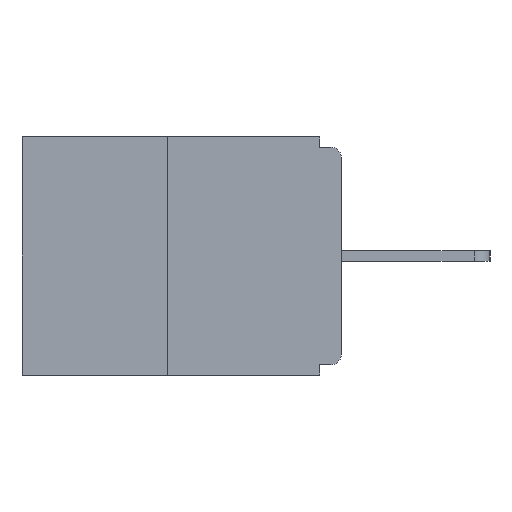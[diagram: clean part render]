
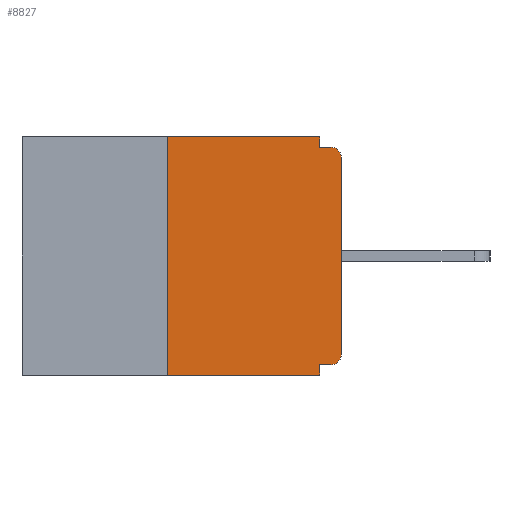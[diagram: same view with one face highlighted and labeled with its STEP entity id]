
A CAD part, left-side view. The second image highlights one B-rep face of the part: STEP entity #8827.
In plain terms, the highlighted planar face has unit normal (-1, 0, 0).
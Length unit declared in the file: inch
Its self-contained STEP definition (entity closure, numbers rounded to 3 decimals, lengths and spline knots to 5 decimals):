
#104 = DIRECTION ( 'NONE',  ( 0., 0., -1. ) ) ;
#195 = CARTESIAN_POINT ( 'NONE',  ( 0., 0.031, -0.343 ) ) ;
#654 = EDGE_CURVE ( 'NONE', #1624, #10731, #8116, .T. ) ;
#824 = EDGE_CURVE ( 'NONE', #11968, #11429, #8155, .T. ) ;
#857 = CARTESIAN_POINT ( 'NONE',  ( 0., 0.46, 0. ) ) ;
#1191 = LINE ( 'NONE', #7887, #2942 ) ;
#1624 = VERTEX_POINT ( 'NONE', #2291 ) ;
#1699 = CARTESIAN_POINT ( 'NONE',  ( 0., 0.031, 0. ) ) ;
#1733 = ORIENTED_EDGE ( 'NONE', *, *, #8710, .T. ) ;
#2024 = DIRECTION ( 'NONE',  ( 0., 0., 1. ) ) ;
#2278 = LINE ( 'NONE', #11873, #8017 ) ;
#2291 = CARTESIAN_POINT ( 'NONE',  ( 0., 0.031, -0.015 ) ) ;
#2858 = DIRECTION ( 'NONE',  ( 0., 0., -1. ) ) ;
#2942 = VECTOR ( 'NONE', #5036, 39.37008 ) ;
#2958 = CARTESIAN_POINT ( 'NONE',  ( 0., 0., -0.015 ) ) ;
#3129 = EDGE_CURVE ( 'NONE', #13975, #12895, #1191, .T. ) ;
#3325 = AXIS2_PLACEMENT_3D ( 'NONE', #9244, #11876, #104 ) ;
#3778 = CARTESIAN_POINT ( 'NONE',  ( 0., 0.015, -0.328 ) ) ;
#3844 = EDGE_CURVE ( 'NONE', #11429, #1624, #8609, .T. ) ;
#4125 = ORIENTED_EDGE ( 'NONE', *, *, #3844, .F. ) ;
#4272 = DIRECTION ( 'NONE',  ( 0., -1., 0. ) ) ;
#4314 = DIRECTION ( 'NONE',  ( 0., -1., 0. ) ) ;
#4321 = LINE ( 'NONE', #195, #10797 ) ;
#4856 = ORIENTED_EDGE ( 'NONE', *, *, #3129, .T. ) ;
#4951 = CIRCLE ( 'NONE', #3325, 0.015 ) ;
#4992 = AXIS2_PLACEMENT_3D ( 'NONE', #12094, #14633, #2858 ) ;
#5036 = DIRECTION ( 'NONE',  ( 0., -1., 0. ) ) ;
#5140 = EDGE_CURVE ( 'NONE', #9505, #16382, #11121, .T. ) ;
#5442 = ORIENTED_EDGE ( 'NONE', *, *, #10091, .F. ) ;
#5775 = DIRECTION ( 'NONE',  ( 0., 0., -1. ) ) ;
#5780 = CARTESIAN_POINT ( 'NONE',  ( 0., 0.25, -0.343 ) ) ;
#5979 = CARTESIAN_POINT ( 'NONE',  ( 0., 0.031, -0.343 ) ) ;
#6184 = ORIENTED_EDGE ( 'NONE', *, *, #6831, .F. ) ;
#6249 = DIRECTION ( 'NONE',  ( 0., 0., 1. ) ) ;
#6585 = VECTOR ( 'NONE', #2024, 39.37008 ) ;
#6831 = EDGE_CURVE ( 'NONE', #7837, #9933, #2278, .T. ) ;
#7065 = CARTESIAN_POINT ( 'NONE',  ( 0., 0.25, 0. ) ) ;
#7837 = VERTEX_POINT ( 'NONE', #3778 ) ;
#7887 = CARTESIAN_POINT ( 'NONE',  ( 0., 0.46, -0.343 ) ) ;
#8017 = VECTOR ( 'NONE', #8023, 39.37008 ) ;
#8023 = DIRECTION ( 'NONE',  ( 0., 1., 0. ) ) ;
#8116 = LINE ( 'NONE', #2958, #9184 ) ;
#8155 = LINE ( 'NONE', #14136, #13614 ) ;
#8609 = LINE ( 'NONE', #15327, #10769 ) ;
#8710 = EDGE_CURVE ( 'NONE', #16382, #10731, #13024, .T. ) ;
#8827 = ADVANCED_FACE ( 'NONE', ( #12708 ), #15400, .F. ) ;
#8839 = CARTESIAN_POINT ( 'NONE',  ( 0., 0.25, 0. ) ) ;
#8859 = ORIENTED_EDGE ( 'NONE', *, *, #654, .F. ) ;
#9184 = VECTOR ( 'NONE', #4314, 39.37008 ) ;
#9244 = CARTESIAN_POINT ( 'NONE',  ( 0., 0.015, -0.313 ) ) ;
#9505 = VERTEX_POINT ( 'NONE', #9589 ) ;
#9589 = CARTESIAN_POINT ( 'NONE',  ( 0., 0., -0.313 ) ) ;
#9782 = ORIENTED_EDGE ( 'NONE', *, *, #11628, .T. ) ;
#9933 = VERTEX_POINT ( 'NONE', #14328 ) ;
#10091 = EDGE_CURVE ( 'NONE', #9933, #12895, #4321, .T. ) ;
#10225 = LINE ( 'NONE', #8839, #13566 ) ;
#10244 = AXIS2_PLACEMENT_3D ( 'NONE', #857, #16616, #11095 ) ;
#10671 = ORIENTED_EDGE ( 'NONE', *, *, #824, .F. ) ;
#10731 = VERTEX_POINT ( 'NONE', #12472 ) ;
#10769 = VECTOR ( 'NONE', #15154, 39.37008 ) ;
#10797 = VECTOR ( 'NONE', #5775, 39.37008 ) ;
#11095 = DIRECTION ( 'NONE',  ( 0., 0., -1. ) ) ;
#11121 = LINE ( 'NONE', #12300, #6585 ) ;
#11316 = ORIENTED_EDGE ( 'NONE', *, *, #5140, .T. ) ;
#11429 = VERTEX_POINT ( 'NONE', #1699 ) ;
#11628 = EDGE_CURVE ( 'NONE', #7837, #9505, #4951, .T. ) ;
#11873 = CARTESIAN_POINT ( 'NONE',  ( 0., 0., -0.328 ) ) ;
#11876 = DIRECTION ( 'NONE',  ( -1., 0., 0. ) ) ;
#11968 = VERTEX_POINT ( 'NONE', #7065 ) ;
#12094 = CARTESIAN_POINT ( 'NONE',  ( 0., 0.015, -0.03 ) ) ;
#12300 = CARTESIAN_POINT ( 'NONE',  ( 0., 0., 0. ) ) ;
#12413 = ORIENTED_EDGE ( 'NONE', *, *, #15120, .F. ) ;
#12472 = CARTESIAN_POINT ( 'NONE',  ( 0., 0.015, -0.015 ) ) ;
#12708 = FACE_OUTER_BOUND ( 'NONE', #14268, .T. ) ;
#12895 = VERTEX_POINT ( 'NONE', #5979 ) ;
#13024 = CIRCLE ( 'NONE', #4992, 0.015 ) ;
#13566 = VECTOR ( 'NONE', #6249, 39.37008 ) ;
#13614 = VECTOR ( 'NONE', #4272, 39.37008 ) ;
#13975 = VERTEX_POINT ( 'NONE', #5780 ) ;
#14136 = CARTESIAN_POINT ( 'NONE',  ( 0., 0.46, 0. ) ) ;
#14268 = EDGE_LOOP ( 'NONE', ( #10671, #12413, #4856, #5442, #6184, #9782, #11316, #1733, #8859, #4125 ) ) ;
#14328 = CARTESIAN_POINT ( 'NONE',  ( 0., 0.031, -0.328 ) ) ;
#14633 = DIRECTION ( 'NONE',  ( -1., 0., 0. ) ) ;
#15120 = EDGE_CURVE ( 'NONE', #13975, #11968, #10225, .T. ) ;
#15154 = DIRECTION ( 'NONE',  ( 0., 0., -1. ) ) ;
#15327 = CARTESIAN_POINT ( 'NONE',  ( 0., 0.031, 0. ) ) ;
#15400 = PLANE ( 'NONE',  #10244 ) ;
#16382 = VERTEX_POINT ( 'NONE', #16704 ) ;
#16616 = DIRECTION ( 'NONE',  ( 1., 0., 0. ) ) ;
#16704 = CARTESIAN_POINT ( 'NONE',  ( 0., 0., -0.03 ) ) ;
